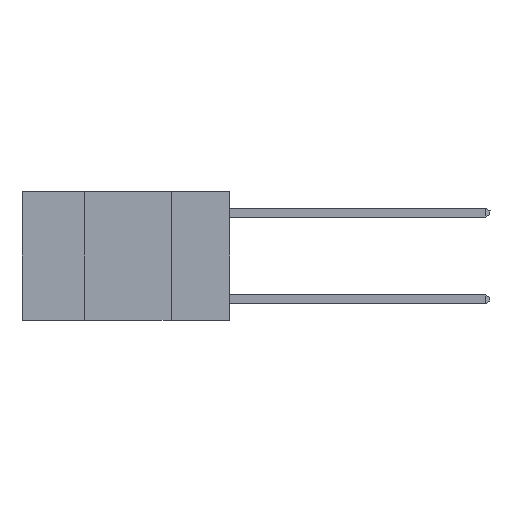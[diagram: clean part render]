
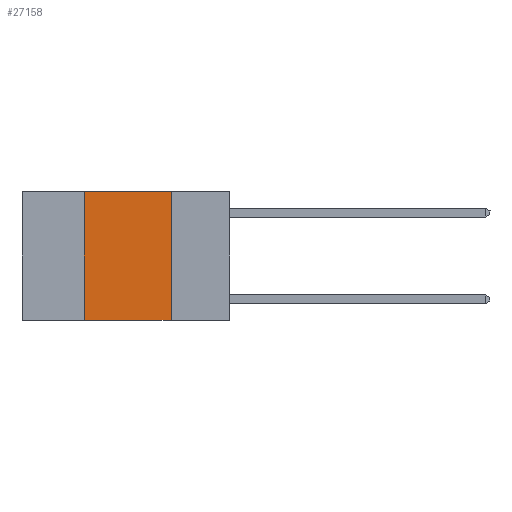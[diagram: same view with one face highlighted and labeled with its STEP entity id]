
A CAD part, left-side view. The second image highlights one B-rep face of the part: STEP entity #27158.
In plain terms, the highlighted planar face has unit normal (-1, 0, 0).
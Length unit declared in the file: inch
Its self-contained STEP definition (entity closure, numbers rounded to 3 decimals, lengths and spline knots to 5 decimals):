
#121 = CARTESIAN_POINT ( 'NONE',  ( 0., 0.17, 0. ) ) ;
#1358 = CARTESIAN_POINT ( 'NONE',  ( 0., 0.42, -0.37 ) ) ;
#1732 = EDGE_LOOP ( 'NONE', ( #23357, #15817, #8036, #21958 ) ) ;
#3070 = VECTOR ( 'NONE', #18987, 39.37008 ) ;
#6534 = EDGE_CURVE ( 'NONE', #30036, #28607, #23861, .T. ) ;
#7334 = CARTESIAN_POINT ( 'NONE',  ( 0., 0.42, 0. ) ) ;
#8036 = ORIENTED_EDGE ( 'NONE', *, *, #29101, .F. ) ;
#8062 = DIRECTION ( 'NONE',  ( 0., 0., 1. ) ) ;
#8412 = DIRECTION ( 'NONE',  ( 1., 0., 0. ) ) ;
#9720 = LINE ( 'NONE', #7334, #28159 ) ;
#10303 = DIRECTION ( 'NONE',  ( 0., -1., 0. ) ) ;
#12348 = EDGE_CURVE ( 'NONE', #25278, #28607, #14503, .T. ) ;
#12856 = DIRECTION ( 'NONE',  ( 0., 0., -1. ) ) ;
#13604 = DIRECTION ( 'NONE',  ( 0., 0., -1. ) ) ;
#14503 = LINE ( 'NONE', #121, #25240 ) ;
#14640 = CARTESIAN_POINT ( 'NONE',  ( 0., 0.17, -0.37 ) ) ;
#15381 = CARTESIAN_POINT ( 'NONE',  ( 0., 0.6, 0. ) ) ;
#15817 = ORIENTED_EDGE ( 'NONE', *, *, #22920, .F. ) ;
#17762 = AXIS2_PLACEMENT_3D ( 'NONE', #15381, #8412, #12856 ) ;
#18987 = DIRECTION ( 'NONE',  ( 0., -1., 0. ) ) ;
#19538 = CARTESIAN_POINT ( 'NONE',  ( 0., 0.17, 0. ) ) ;
#19766 = LINE ( 'NONE', #22270, #22139 ) ;
#20266 = FACE_OUTER_BOUND ( 'NONE', #1732, .T. ) ;
#21958 = ORIENTED_EDGE ( 'NONE', *, *, #6534, .T. ) ;
#22139 = VECTOR ( 'NONE', #10303, 39.37008 ) ;
#22270 = CARTESIAN_POINT ( 'NONE',  ( 0., 0.6, 0. ) ) ;
#22920 = EDGE_CURVE ( 'NONE', #25570, #25278, #19766, .T. ) ;
#23357 = ORIENTED_EDGE ( 'NONE', *, *, #12348, .F. ) ;
#23552 = CARTESIAN_POINT ( 'NONE',  ( 0., 0.6, -0.37 ) ) ;
#23861 = LINE ( 'NONE', #23552, #3070 ) ;
#24835 = PLANE ( 'NONE',  #17762 ) ;
#25240 = VECTOR ( 'NONE', #13604, 39.37008 ) ;
#25278 = VERTEX_POINT ( 'NONE', #19538 ) ;
#25570 = VERTEX_POINT ( 'NONE', #26123 ) ;
#26123 = CARTESIAN_POINT ( 'NONE',  ( 0., 0.42, 0. ) ) ;
#27158 = ADVANCED_FACE ( 'NONE', ( #20266 ), #24835, .F. ) ;
#28159 = VECTOR ( 'NONE', #8062, 39.37008 ) ;
#28607 = VERTEX_POINT ( 'NONE', #14640 ) ;
#29101 = EDGE_CURVE ( 'NONE', #30036, #25570, #9720, .T. ) ;
#30036 = VERTEX_POINT ( 'NONE', #1358 ) ;
